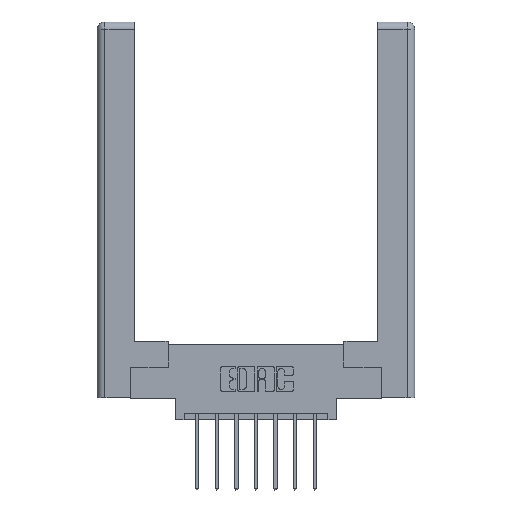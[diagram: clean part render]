
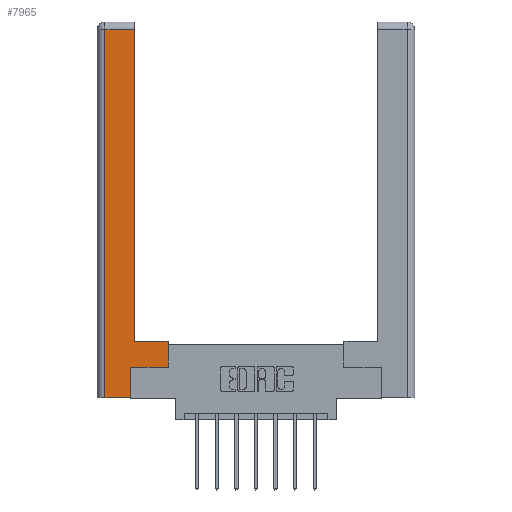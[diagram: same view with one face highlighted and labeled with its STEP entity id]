
A CAD part, top view. The second image highlights one B-rep face of the part: STEP entity #7965.
In plain terms, the highlighted planar face has unit normal (0, 0, 1).
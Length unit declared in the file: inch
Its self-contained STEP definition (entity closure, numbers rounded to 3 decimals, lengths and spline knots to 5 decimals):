
#282 = ORIENTED_EDGE ( 'NONE', *, *, #11520, .T. ) ;
#566 = LINE ( 'NONE', #2582, #717 ) ;
#661 = EDGE_CURVE ( 'NONE', #2034, #3239, #4565, .T. ) ;
#681 = PLANE ( 'NONE',  #5494 ) ;
#717 = VECTOR ( 'NONE', #12260, 39.37008 ) ;
#725 = ORIENTED_EDGE ( 'NONE', *, *, #7145, .T. ) ;
#761 = LINE ( 'NONE', #12543, #12165 ) ;
#1138 = CARTESIAN_POINT ( 'NONE',  ( 0.265, 0.245, 0. ) ) ;
#1152 = ORIENTED_EDGE ( 'NONE', *, *, #10020, .T. ) ;
#1358 = EDGE_CURVE ( 'NONE', #2070, #9672, #6578, .T. ) ;
#1374 = VECTOR ( 'NONE', #9474, 39.37008 ) ;
#1461 = ORIENTED_EDGE ( 'NONE', *, *, #661, .T. ) ;
#1514 = VERTEX_POINT ( 'NONE', #4736 ) ;
#1618 = DIRECTION ( 'NONE',  ( 0., -1., 0. ) ) ;
#1914 = CARTESIAN_POINT ( 'NONE',  ( 0.565, 0.45, 0. ) ) ;
#1936 = LINE ( 'NONE', #1914, #7330 ) ;
#1974 = ORIENTED_EDGE ( 'NONE', *, *, #10306, .T. ) ;
#2034 = VERTEX_POINT ( 'NONE', #4983 ) ;
#2070 = VERTEX_POINT ( 'NONE', #1138 ) ;
#2145 = ORIENTED_EDGE ( 'NONE', *, *, #7614, .T. ) ;
#2413 = EDGE_CURVE ( 'NONE', #9672, #7623, #1936, .T. ) ;
#2582 = CARTESIAN_POINT ( 'NONE',  ( 0.295, 3., 0. ) ) ;
#2638 = LINE ( 'NONE', #4909, #4045 ) ;
#2915 = CARTESIAN_POINT ( 'NONE',  ( 0.565, 0.245, 0. ) ) ;
#3239 = VERTEX_POINT ( 'NONE', #5560 ) ;
#3272 = LINE ( 'NONE', #3396, #12371 ) ;
#3320 = CARTESIAN_POINT ( 'NONE',  ( 0.565, 0.45, 0. ) ) ;
#3396 = CARTESIAN_POINT ( 'NONE',  ( 0.265, 0.245, 0. ) ) ;
#3400 = VERTEX_POINT ( 'NONE', #12654 ) ;
#4045 = VECTOR ( 'NONE', #10837, 39.37008 ) ;
#4101 = VECTOR ( 'NONE', #11421, 39.37008 ) ;
#4445 = CARTESIAN_POINT ( 'NONE',  ( 0.0615, 0., 0. ) ) ;
#4565 = LINE ( 'NONE', #4445, #9200 ) ;
#4736 = CARTESIAN_POINT ( 'NONE',  ( 0.295, 2.94, 0. ) ) ;
#4909 = CARTESIAN_POINT ( 'NONE',  ( 0.295, 0.45, 0. ) ) ;
#4983 = CARTESIAN_POINT ( 'NONE',  ( 0.0615, 2.94, 0. ) ) ;
#5494 = AXIS2_PLACEMENT_3D ( 'NONE', #10572, #7654, #7611 ) ;
#5560 = CARTESIAN_POINT ( 'NONE',  ( 0.0615, 0., 0. ) ) ;
#5789 = DIRECTION ( 'NONE',  ( 0., 1., 0. ) ) ;
#6327 = ORIENTED_EDGE ( 'NONE', *, *, #1358, .T. ) ;
#6531 = CARTESIAN_POINT ( 'NONE',  ( 0.565, 0.245, 0. ) ) ;
#6578 = LINE ( 'NONE', #6531, #4101 ) ;
#7145 = EDGE_CURVE ( 'NONE', #7623, #3400, #2638, .T. ) ;
#7330 = VECTOR ( 'NONE', #5789, 39.37008 ) ;
#7611 = DIRECTION ( 'NONE',  ( -1., 0., 0. ) ) ;
#7614 = EDGE_CURVE ( 'NONE', #12085, #2070, #3272, .T. ) ;
#7623 = VERTEX_POINT ( 'NONE', #3320 ) ;
#7654 = DIRECTION ( 'NONE',  ( 0., 0., -1. ) ) ;
#7965 = ADVANCED_FACE ( 'NONE', ( #8230 ), #681, .F. ) ;
#8230 = FACE_OUTER_BOUND ( 'NONE', #8542, .T. ) ;
#8542 = EDGE_LOOP ( 'NONE', ( #282, #1152, #1461, #1974, #2145, #6327, #11360, #725 ) ) ;
#9200 = VECTOR ( 'NONE', #1618, 39.37008 ) ;
#9389 = CARTESIAN_POINT ( 'NONE',  ( 0.265, 0., 0. ) ) ;
#9474 = DIRECTION ( 'NONE',  ( 1., 0., 0. ) ) ;
#9672 = VERTEX_POINT ( 'NONE', #2915 ) ;
#10020 = EDGE_CURVE ( 'NONE', #1514, #2034, #761, .T. ) ;
#10306 = EDGE_CURVE ( 'NONE', #3239, #12085, #11071, .T. ) ;
#10572 = CARTESIAN_POINT ( 'NONE',  ( 0., 0., 0. ) ) ;
#10837 = DIRECTION ( 'NONE',  ( -1., 0., 0. ) ) ;
#11063 = CARTESIAN_POINT ( 'NONE',  ( 0.265, 0., 0. ) ) ;
#11071 = LINE ( 'NONE', #9389, #1374 ) ;
#11170 = DIRECTION ( 'NONE',  ( 0., 1., 0. ) ) ;
#11360 = ORIENTED_EDGE ( 'NONE', *, *, #2413, .T. ) ;
#11421 = DIRECTION ( 'NONE',  ( 1., 0., 0. ) ) ;
#11520 = EDGE_CURVE ( 'NONE', #3400, #1514, #566, .T. ) ;
#12085 = VERTEX_POINT ( 'NONE', #11063 ) ;
#12165 = VECTOR ( 'NONE', #12416, 39.37008 ) ;
#12260 = DIRECTION ( 'NONE',  ( 0., 1., 0. ) ) ;
#12371 = VECTOR ( 'NONE', #11170, 39.37008 ) ;
#12416 = DIRECTION ( 'NONE',  ( -1., 0., 0. ) ) ;
#12543 = CARTESIAN_POINT ( 'NONE',  ( 0.0615, 2.94, 0. ) ) ;
#12654 = CARTESIAN_POINT ( 'NONE',  ( 0.295, 0.45, 0. ) ) ;
